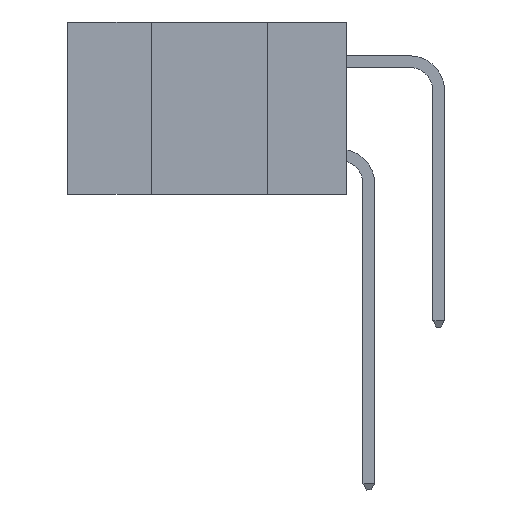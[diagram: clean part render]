
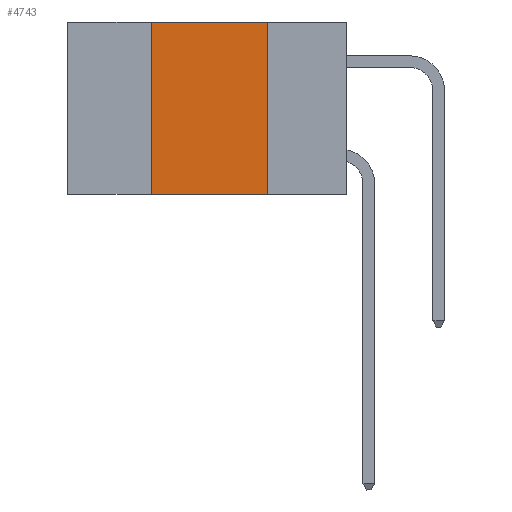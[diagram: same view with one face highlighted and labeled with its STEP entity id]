
A CAD part, left-side view. The second image highlights one B-rep face of the part: STEP entity #4743.
In plain terms, the highlighted planar face has unit normal (-1, 0, 0).
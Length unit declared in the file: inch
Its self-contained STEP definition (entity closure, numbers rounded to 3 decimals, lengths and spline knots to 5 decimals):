
#595 = DIRECTION ( 'NONE',  ( 0., -1., 0. ) ) ;
#994 = DIRECTION ( 'NONE',  ( 0., -1., 0. ) ) ;
#1175 = CARTESIAN_POINT ( 'NONE',  ( 0., 0.42, 0. ) ) ;
#1248 = EDGE_CURVE ( 'NONE', #4839, #7286, #9623, .T. ) ;
#1292 = VECTOR ( 'NONE', #595, 39.37008 ) ;
#1436 = FACE_OUTER_BOUND ( 'NONE', #1738, .T. ) ;
#1738 = EDGE_LOOP ( 'NONE', ( #10110, #2636, #8231, #3360 ) ) ;
#2636 = ORIENTED_EDGE ( 'NONE', *, *, #1248, .F. ) ;
#2837 = LINE ( 'NONE', #6226, #1292 ) ;
#3176 = AXIS2_PLACEMENT_3D ( 'NONE', #7656, #3402, #5871 ) ;
#3360 = ORIENTED_EDGE ( 'NONE', *, *, #5387, .T. ) ;
#3402 = DIRECTION ( 'NONE',  ( 1., 0., 0. ) ) ;
#4416 = DIRECTION ( 'NONE',  ( 0., 0., 1. ) ) ;
#4743 = ADVANCED_FACE ( 'NONE', ( #1436 ), #5162, .F. ) ;
#4750 = CARTESIAN_POINT ( 'NONE',  ( 0., 0.42, 0. ) ) ;
#4839 = VERTEX_POINT ( 'NONE', #4750 ) ;
#5162 = PLANE ( 'NONE',  #3176 ) ;
#5387 = EDGE_CURVE ( 'NONE', #5634, #6793, #2837, .T. ) ;
#5403 = CARTESIAN_POINT ( 'NONE',  ( 0., 0.42, -0.37 ) ) ;
#5634 = VERTEX_POINT ( 'NONE', #5403 ) ;
#5871 = DIRECTION ( 'NONE',  ( 0., 0., -1. ) ) ;
#5960 = LINE ( 'NONE', #1175, #9198 ) ;
#6226 = CARTESIAN_POINT ( 'NONE',  ( 0., 0.6, -0.37 ) ) ;
#6410 = CARTESIAN_POINT ( 'NONE',  ( 0., 0.17, 0. ) ) ;
#6793 = VERTEX_POINT ( 'NONE', #9329 ) ;
#6936 = VECTOR ( 'NONE', #7353, 39.37008 ) ;
#7276 = CARTESIAN_POINT ( 'NONE',  ( 0., 0.17, 0. ) ) ;
#7286 = VERTEX_POINT ( 'NONE', #6410 ) ;
#7353 = DIRECTION ( 'NONE',  ( 0., 0., -1. ) ) ;
#7357 = EDGE_CURVE ( 'NONE', #7286, #6793, #9008, .T. ) ;
#7656 = CARTESIAN_POINT ( 'NONE',  ( 0., 0.6, 0. ) ) ;
#8231 = ORIENTED_EDGE ( 'NONE', *, *, #10664, .F. ) ;
#9008 = LINE ( 'NONE', #7276, #6936 ) ;
#9198 = VECTOR ( 'NONE', #4416, 39.37008 ) ;
#9248 = CARTESIAN_POINT ( 'NONE',  ( 0., 0.6, 0. ) ) ;
#9329 = CARTESIAN_POINT ( 'NONE',  ( 0., 0.17, -0.37 ) ) ;
#9623 = LINE ( 'NONE', #9248, #10415 ) ;
#10110 = ORIENTED_EDGE ( 'NONE', *, *, #7357, .F. ) ;
#10415 = VECTOR ( 'NONE', #994, 39.37008 ) ;
#10664 = EDGE_CURVE ( 'NONE', #5634, #4839, #5960, .T. ) ;
